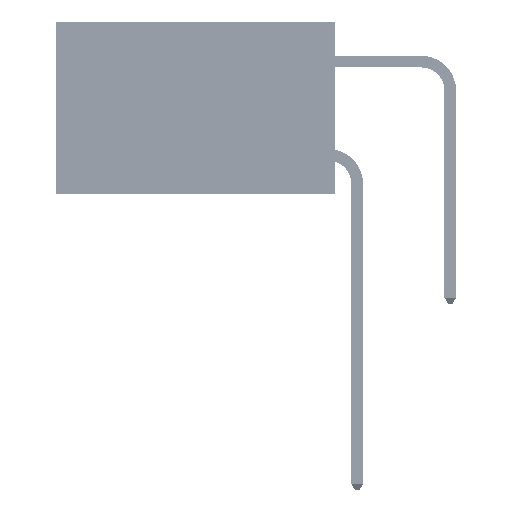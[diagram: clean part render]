
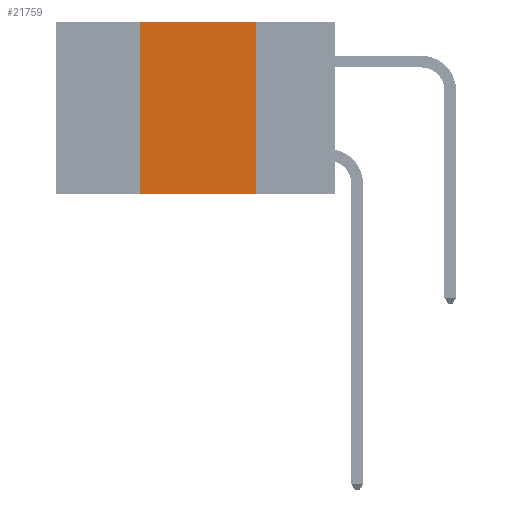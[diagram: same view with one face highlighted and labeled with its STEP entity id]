
A CAD part, left-side view. The second image highlights one B-rep face of the part: STEP entity #21759.
In plain terms, the highlighted planar face has unit normal (-1, 0, 0).
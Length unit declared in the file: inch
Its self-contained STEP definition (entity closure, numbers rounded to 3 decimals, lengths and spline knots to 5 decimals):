
#87 = DIRECTION ( 'NONE',  ( 0., 0., 1. ) ) ;
#355 = EDGE_CURVE ( 'NONE', #1100, #26471, #1767, .T. ) ;
#1100 = VERTEX_POINT ( 'NONE', #24764 ) ;
#1212 = PLANE ( 'NONE',  #35915 ) ;
#1767 = LINE ( 'NONE', #5935, #19785 ) ;
#2106 = EDGE_CURVE ( 'NONE', #40583, #26471, #41997, .T. ) ;
#2343 = DIRECTION ( 'NONE',  ( 0., -1., 0. ) ) ;
#2713 = VECTOR ( 'NONE', #39713, 39.37008 ) ;
#4828 = DIRECTION ( 'NONE',  ( 0., 0., -1. ) ) ;
#5935 = CARTESIAN_POINT ( 'NONE',  ( 0., 0.6, -0.37 ) ) ;
#9955 = CARTESIAN_POINT ( 'NONE',  ( 0., 0.42, 0. ) ) ;
#11680 = VERTEX_POINT ( 'NONE', #9955 ) ;
#12279 = LINE ( 'NONE', #36099, #2713 ) ;
#13386 = VECTOR ( 'NONE', #87, 39.37008 ) ;
#13870 = EDGE_CURVE ( 'NONE', #11680, #40583, #12279, .T. ) ;
#15135 = DIRECTION ( 'NONE',  ( 0., 0., -1. ) ) ;
#16118 = ORIENTED_EDGE ( 'NONE', *, *, #36094, .F. ) ;
#19785 = VECTOR ( 'NONE', #2343, 39.37008 ) ;
#20738 = VECTOR ( 'NONE', #15135, 39.37008 ) ;
#21759 = ADVANCED_FACE ( 'NONE', ( #23623 ), #1212, .F. ) ;
#22903 = ORIENTED_EDGE ( 'NONE', *, *, #355, .T. ) ;
#23077 = CARTESIAN_POINT ( 'NONE',  ( 0., 0.17, 0. ) ) ;
#23623 = FACE_OUTER_BOUND ( 'NONE', #28227, .T. ) ;
#24764 = CARTESIAN_POINT ( 'NONE',  ( 0., 0.42, -0.37 ) ) ;
#26346 = DIRECTION ( 'NONE',  ( 1., 0., 0. ) ) ;
#26471 = VERTEX_POINT ( 'NONE', #37175 ) ;
#28227 = EDGE_LOOP ( 'NONE', ( #32257, #30068, #16118, #22903 ) ) ;
#30068 = ORIENTED_EDGE ( 'NONE', *, *, #13870, .F. ) ;
#32257 = ORIENTED_EDGE ( 'NONE', *, *, #2106, .F. ) ;
#32421 = LINE ( 'NONE', #43062, #13386 ) ;
#32984 = CARTESIAN_POINT ( 'NONE',  ( 0., 0.17, 0. ) ) ;
#35915 = AXIS2_PLACEMENT_3D ( 'NONE', #44188, #26346, #4828 ) ;
#36094 = EDGE_CURVE ( 'NONE', #1100, #11680, #32421, .T. ) ;
#36099 = CARTESIAN_POINT ( 'NONE',  ( 0., 0.6, 0. ) ) ;
#37175 = CARTESIAN_POINT ( 'NONE',  ( 0., 0.17, -0.37 ) ) ;
#39713 = DIRECTION ( 'NONE',  ( 0., -1., 0. ) ) ;
#40583 = VERTEX_POINT ( 'NONE', #23077 ) ;
#41997 = LINE ( 'NONE', #32984, #20738 ) ;
#43062 = CARTESIAN_POINT ( 'NONE',  ( 0., 0.42, 0. ) ) ;
#44188 = CARTESIAN_POINT ( 'NONE',  ( 0., 0.6, 0. ) ) ;
